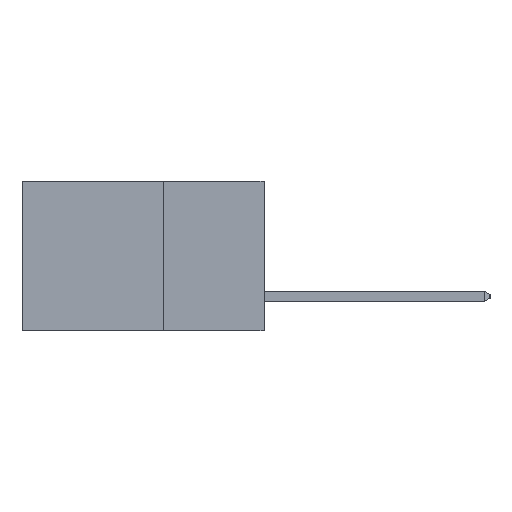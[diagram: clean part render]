
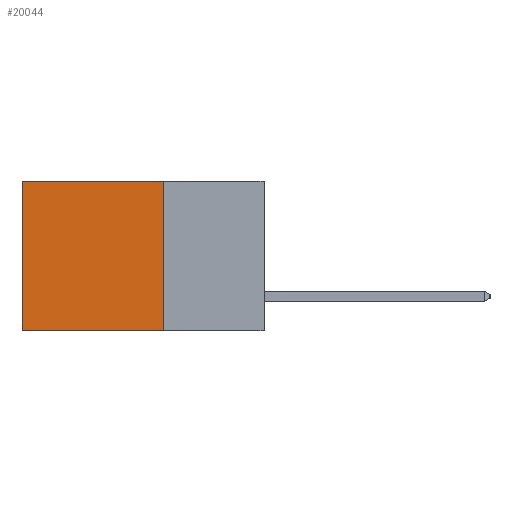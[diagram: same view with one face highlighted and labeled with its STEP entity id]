
A CAD part, left-side view. The second image highlights one B-rep face of the part: STEP entity #20044.
In plain terms, the highlighted planar face has unit normal (-1, 0, 0).
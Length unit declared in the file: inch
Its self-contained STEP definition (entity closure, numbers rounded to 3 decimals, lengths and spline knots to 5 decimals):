
#652 = ORIENTED_EDGE ( 'NONE', *, *, #4622, .T. ) ;
#694 = CARTESIAN_POINT ( 'NONE',  ( 0.2615, 0.25, -0.37 ) ) ;
#1049 = VECTOR ( 'NONE', #8421, 39.37008 ) ;
#2029 = CARTESIAN_POINT ( 'NONE',  ( 0.2615, 0.6, -0.37 ) ) ;
#2239 = DIRECTION ( 'NONE',  ( 0., 0., -1. ) ) ;
#3682 = LINE ( 'NONE', #10908, #19088 ) ;
#4019 = PLANE ( 'NONE',  #16662 ) ;
#4166 = CARTESIAN_POINT ( 'NONE',  ( 0.2615, 0.25, 0. ) ) ;
#4622 = EDGE_CURVE ( 'NONE', #9396, #7158, #15732, .T. ) ;
#5466 = EDGE_CURVE ( 'NONE', #8905, #7158, #3682, .T. ) ;
#6249 = CARTESIAN_POINT ( 'NONE',  ( 0.2615, 0.6, 0. ) ) ;
#6812 = CARTESIAN_POINT ( 'NONE',  ( 0.2615, 0.25, 0. ) ) ;
#7158 = VERTEX_POINT ( 'NONE', #2029 ) ;
#7188 = DIRECTION ( 'NONE',  ( 1., 0., 0. ) ) ;
#7718 = VERTEX_POINT ( 'NONE', #4166 ) ;
#7891 = DIRECTION ( 'NONE',  ( 0., 0., -1. ) ) ;
#7999 = VECTOR ( 'NONE', #7891, 39.37008 ) ;
#8421 = DIRECTION ( 'NONE',  ( 0., 1., 0. ) ) ;
#8905 = VERTEX_POINT ( 'NONE', #10497 ) ;
#9396 = VERTEX_POINT ( 'NONE', #6249 ) ;
#9587 = LINE ( 'NONE', #6812, #1049 ) ;
#10497 = CARTESIAN_POINT ( 'NONE',  ( 0.2615, 0.25, -0.37 ) ) ;
#10908 = CARTESIAN_POINT ( 'NONE',  ( 0.2615, 0.25, -0.37 ) ) ;
#11011 = DIRECTION ( 'NONE',  ( 0., 1., 0. ) ) ;
#14594 = FACE_OUTER_BOUND ( 'NONE', #17814, .T. ) ;
#14759 = ORIENTED_EDGE ( 'NONE', *, *, #18060, .T. ) ;
#15500 = ORIENTED_EDGE ( 'NONE', *, *, #5466, .F. ) ;
#15557 = ORIENTED_EDGE ( 'NONE', *, *, #15632, .F. ) ;
#15632 = EDGE_CURVE ( 'NONE', #7718, #8905, #19588, .T. ) ;
#15732 = LINE ( 'NONE', #17122, #7999 ) ;
#16662 = AXIS2_PLACEMENT_3D ( 'NONE', #694, #7188, #17960 ) ;
#17122 = CARTESIAN_POINT ( 'NONE',  ( 0.2615, 0.6, -0.37 ) ) ;
#17773 = CARTESIAN_POINT ( 'NONE',  ( 0.2615, 0.25, -0.37 ) ) ;
#17814 = EDGE_LOOP ( 'NONE', ( #652, #15500, #15557, #14759 ) ) ;
#17960 = DIRECTION ( 'NONE',  ( 0., 0., -1. ) ) ;
#18060 = EDGE_CURVE ( 'NONE', #7718, #9396, #9587, .T. ) ;
#19088 = VECTOR ( 'NONE', #11011, 39.37008 ) ;
#19145 = VECTOR ( 'NONE', #2239, 39.37008 ) ;
#19588 = LINE ( 'NONE', #17773, #19145 ) ;
#20044 = ADVANCED_FACE ( 'NONE', ( #14594 ), #4019, .F. ) ;
